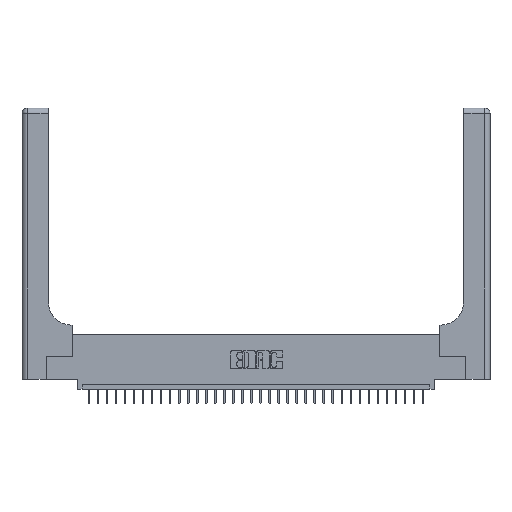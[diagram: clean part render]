
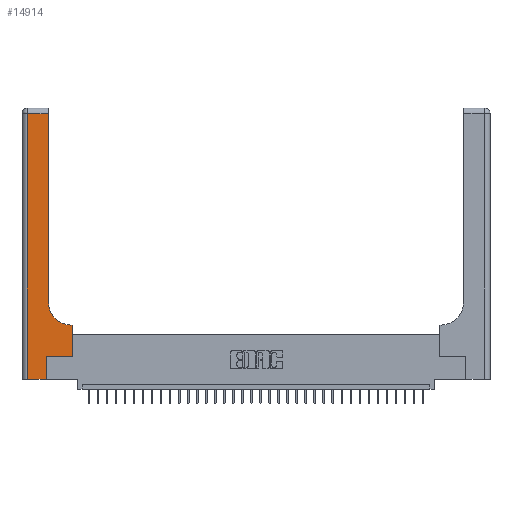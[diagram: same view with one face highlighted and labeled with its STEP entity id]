
A CAD part, top view. The second image highlights one B-rep face of the part: STEP entity #14914.
In plain terms, the highlighted planar face has unit normal (0, 0, 1).
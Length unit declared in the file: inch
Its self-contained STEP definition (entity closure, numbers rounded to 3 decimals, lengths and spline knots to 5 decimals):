
#752 = CARTESIAN_POINT ( 'NONE',  ( 0.5415, 0.6, 0.37 ) ) ;
#1468 = CARTESIAN_POINT ( 'NONE',  ( 0.5585, 0.25, 0.37 ) ) ;
#1765 = EDGE_CURVE ( 'NONE', #8234, #24222, #9722, .T. ) ;
#1870 = VERTEX_POINT ( 'NONE', #17527 ) ;
#2180 = EDGE_CURVE ( 'NONE', #28690, #9464, #5920, .T. ) ;
#2858 = DIRECTION ( 'NONE',  ( 0., -1., 0. ) ) ;
#3049 = ORIENTED_EDGE ( 'NONE', *, *, #2180, .T. ) ;
#3202 = DIRECTION ( 'NONE',  ( 1., 0., 0. ) ) ;
#3586 = VECTOR ( 'NONE', #15347, 39.37008 ) ;
#4053 = CARTESIAN_POINT ( 'NONE',  ( 0., 0., 0.37 ) ) ;
#5766 = DIRECTION ( 'NONE',  ( 0., 1., 0. ) ) ;
#5920 = LINE ( 'NONE', #16034, #33442 ) ;
#6745 = CARTESIAN_POINT ( 'NONE',  ( 0.2915, 0.6, 0.37 ) ) ;
#6993 = CIRCLE ( 'NONE', #11296, 0.25 ) ;
#7732 = CARTESIAN_POINT ( 'NONE',  ( 0.5585, 0.25, 0.37 ) ) ;
#7760 = CARTESIAN_POINT ( 'NONE',  ( 0.269, 0., 0.37 ) ) ;
#8234 = VERTEX_POINT ( 'NONE', #16753 ) ;
#8336 = VERTEX_POINT ( 'NONE', #14547 ) ;
#8629 = LINE ( 'NONE', #7760, #3586 ) ;
#9464 = VERTEX_POINT ( 'NONE', #29801 ) ;
#9722 = LINE ( 'NONE', #6745, #20575 ) ;
#11296 = AXIS2_PLACEMENT_3D ( 'NONE', #26364, #34366, #15621 ) ;
#11420 = EDGE_CURVE ( 'NONE', #1870, #19587, #32145, .T. ) ;
#12209 = ORIENTED_EDGE ( 'NONE', *, *, #1765, .T. ) ;
#12256 = EDGE_LOOP ( 'NONE', ( #3049, #25515, #27209, #29151, #16237, #18632, #33922, #12209, #31517 ) ) ;
#12381 = DIRECTION ( 'NONE',  ( 1., 0., 0. ) ) ;
#12575 = AXIS2_PLACEMENT_3D ( 'NONE', #17136, #27853, #22635 ) ;
#13194 = VECTOR ( 'NONE', #26513, 39.37008 ) ;
#14547 = CARTESIAN_POINT ( 'NONE',  ( 0.06, 2.94, 0.37 ) ) ;
#14914 = ADVANCED_FACE ( 'NONE', ( #28083 ), #24950, .F. ) ;
#15347 = DIRECTION ( 'NONE',  ( 0., 1., 0. ) ) ;
#15621 = DIRECTION ( 'NONE',  ( 1., 0., 0. ) ) ;
#15987 = DIRECTION ( 'NONE',  ( 0., 1., 0. ) ) ;
#16034 = CARTESIAN_POINT ( 'NONE',  ( 0.2915, 3., 0.37 ) ) ;
#16237 = ORIENTED_EDGE ( 'NONE', *, *, #19120, .T. ) ;
#16505 = VECTOR ( 'NONE', #15987, 39.37008 ) ;
#16753 = CARTESIAN_POINT ( 'NONE',  ( 0.5585, 0.6, 0.37 ) ) ;
#17136 = CARTESIAN_POINT ( 'NONE',  ( 0., 3., 0.37 ) ) ;
#17527 = CARTESIAN_POINT ( 'NONE',  ( 0.06, 0., 0.37 ) ) ;
#17764 = LINE ( 'NONE', #7732, #16505 ) ;
#18632 = ORIENTED_EDGE ( 'NONE', *, *, #31775, .T. ) ;
#19120 = EDGE_CURVE ( 'NONE', #19587, #27482, #8629, .T. ) ;
#19587 = VERTEX_POINT ( 'NONE', #31046 ) ;
#20575 = VECTOR ( 'NONE', #31101, 39.37008 ) ;
#20629 = EDGE_CURVE ( 'NONE', #24222, #28690, #6993, .T. ) ;
#21882 = EDGE_CURVE ( 'NONE', #28065, #8234, #17764, .T. ) ;
#22039 = EDGE_CURVE ( 'NONE', #9464, #8336, #34432, .T. ) ;
#22144 = CARTESIAN_POINT ( 'NONE',  ( 0.269, 0.25, 0.37 ) ) ;
#22429 = VECTOR ( 'NONE', #2858, 39.37008 ) ;
#22635 = DIRECTION ( 'NONE',  ( -1., 0., 0. ) ) ;
#24222 = VERTEX_POINT ( 'NONE', #752 ) ;
#24890 = LINE ( 'NONE', #22144, #25745 ) ;
#24950 = PLANE ( 'NONE',  #12575 ) ;
#25515 = ORIENTED_EDGE ( 'NONE', *, *, #22039, .T. ) ;
#25745 = VECTOR ( 'NONE', #3202, 39.37008 ) ;
#25913 = VECTOR ( 'NONE', #12381, 39.37008 ) ;
#26364 = CARTESIAN_POINT ( 'NONE',  ( 0.5415, 0.85, 0.37 ) ) ;
#26513 = DIRECTION ( 'NONE',  ( -1., 0., 0. ) ) ;
#27209 = ORIENTED_EDGE ( 'NONE', *, *, #33665, .T. ) ;
#27354 = CARTESIAN_POINT ( 'NONE',  ( 0.06, 3., 0.37 ) ) ;
#27482 = VERTEX_POINT ( 'NONE', #34070 ) ;
#27853 = DIRECTION ( 'NONE',  ( 0., 0., -1. ) ) ;
#28065 = VERTEX_POINT ( 'NONE', #1468 ) ;
#28083 = FACE_OUTER_BOUND ( 'NONE', #12256, .T. ) ;
#28690 = VERTEX_POINT ( 'NONE', #30527 ) ;
#29151 = ORIENTED_EDGE ( 'NONE', *, *, #11420, .T. ) ;
#29302 = CARTESIAN_POINT ( 'NONE',  ( 0., 2.94, 0.37 ) ) ;
#29801 = CARTESIAN_POINT ( 'NONE',  ( 0.2915, 2.94, 0.37 ) ) ;
#30527 = CARTESIAN_POINT ( 'NONE',  ( 0.2915, 0.85, 0.37 ) ) ;
#30762 = LINE ( 'NONE', #27354, #22429 ) ;
#31046 = CARTESIAN_POINT ( 'NONE',  ( 0.269, 0., 0.37 ) ) ;
#31101 = DIRECTION ( 'NONE',  ( -1., 0., 0. ) ) ;
#31517 = ORIENTED_EDGE ( 'NONE', *, *, #20629, .T. ) ;
#31775 = EDGE_CURVE ( 'NONE', #27482, #28065, #24890, .T. ) ;
#32145 = LINE ( 'NONE', #4053, #25913 ) ;
#33442 = VECTOR ( 'NONE', #5766, 39.37008 ) ;
#33665 = EDGE_CURVE ( 'NONE', #8336, #1870, #30762, .T. ) ;
#33922 = ORIENTED_EDGE ( 'NONE', *, *, #21882, .T. ) ;
#34070 = CARTESIAN_POINT ( 'NONE',  ( 0.269, 0.25, 0.37 ) ) ;
#34366 = DIRECTION ( 'NONE',  ( 0., 0., -1. ) ) ;
#34432 = LINE ( 'NONE', #29302, #13194 ) ;
